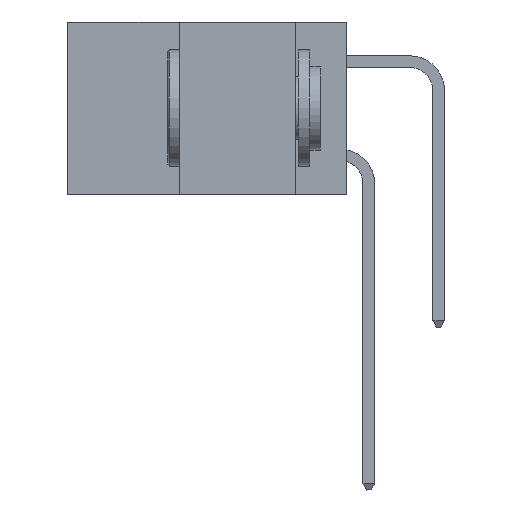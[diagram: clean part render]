
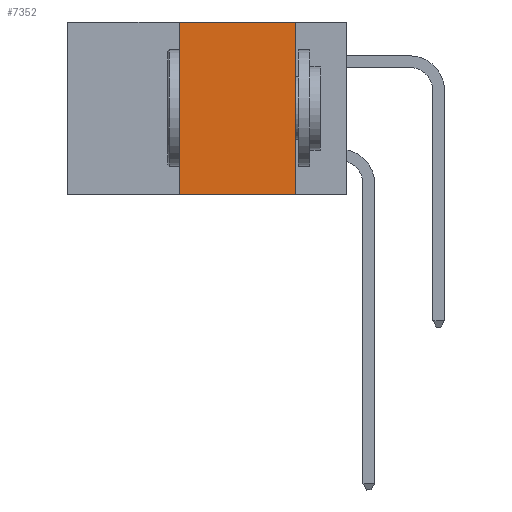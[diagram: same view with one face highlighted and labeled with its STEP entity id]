
A CAD part, left-side view. The second image highlights one B-rep face of the part: STEP entity #7352.
In plain terms, the highlighted planar face has unit normal (-1, 0, 0).
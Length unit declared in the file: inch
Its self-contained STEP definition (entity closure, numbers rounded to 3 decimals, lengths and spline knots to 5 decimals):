
#1701 = DIRECTION ( 'NONE',  ( 1., 0., 0. ) ) ;
#2170 = VERTEX_POINT ( 'NONE', #22658 ) ;
#2224 = ORIENTED_EDGE ( 'NONE', *, *, #2939, .T. ) ;
#2939 = EDGE_CURVE ( 'NONE', #2170, #36981, #4788, .T. ) ;
#4088 = CARTESIAN_POINT ( 'NONE',  ( 0., 0.6, 0. ) ) ;
#4305 = CARTESIAN_POINT ( 'NONE',  ( 0., 0.11, -0.37 ) ) ;
#4788 = LINE ( 'NONE', #7732, #15720 ) ;
#5493 = EDGE_CURVE ( 'NONE', #2170, #9404, #33022, .T. ) ;
#5904 = LINE ( 'NONE', #30891, #37155 ) ;
#6546 = EDGE_CURVE ( 'NONE', #9404, #38411, #5904, .T. ) ;
#6867 = CARTESIAN_POINT ( 'NONE',  ( 0., 0.11, 0. ) ) ;
#6978 = VECTOR ( 'NONE', #37187, 39.37008 ) ;
#7010 = DIRECTION ( 'NONE',  ( 0., -1., 0. ) ) ;
#7352 = ADVANCED_FACE ( 'NONE', ( #10082 ), #16907, .F. ) ;
#7423 = VECTOR ( 'NONE', #21959, 39.37008 ) ;
#7446 = CARTESIAN_POINT ( 'NONE',  ( 0., 0.36, 0. ) ) ;
#7732 = CARTESIAN_POINT ( 'NONE',  ( 0., 0.6, -0.37 ) ) ;
#9404 = VERTEX_POINT ( 'NONE', #7446 ) ;
#10082 = FACE_OUTER_BOUND ( 'NONE', #25897, .T. ) ;
#13397 = ORIENTED_EDGE ( 'NONE', *, *, #6546, .F. ) ;
#15720 = VECTOR ( 'NONE', #28938, 39.37008 ) ;
#16907 = PLANE ( 'NONE',  #35026 ) ;
#17008 = LINE ( 'NONE', #6867, #6978 ) ;
#17146 = CARTESIAN_POINT ( 'NONE',  ( 0., 0.11, 0. ) ) ;
#18206 = ORIENTED_EDGE ( 'NONE', *, *, #27128, .F. ) ;
#21959 = DIRECTION ( 'NONE',  ( 0., 0., 1. ) ) ;
#22658 = CARTESIAN_POINT ( 'NONE',  ( 0., 0.36, -0.37 ) ) ;
#25897 = EDGE_LOOP ( 'NONE', ( #18206, #13397, #25953, #2224 ) ) ;
#25953 = ORIENTED_EDGE ( 'NONE', *, *, #5493, .F. ) ;
#27128 = EDGE_CURVE ( 'NONE', #38411, #36981, #17008, .T. ) ;
#28938 = DIRECTION ( 'NONE',  ( 0., -1., 0. ) ) ;
#30891 = CARTESIAN_POINT ( 'NONE',  ( 0., 0.6, 0. ) ) ;
#33022 = LINE ( 'NONE', #34393, #7423 ) ;
#34393 = CARTESIAN_POINT ( 'NONE',  ( 0., 0.36, 0. ) ) ;
#35026 = AXIS2_PLACEMENT_3D ( 'NONE', #4088, #1701, #38776 ) ;
#36981 = VERTEX_POINT ( 'NONE', #4305 ) ;
#37155 = VECTOR ( 'NONE', #7010, 39.37008 ) ;
#37187 = DIRECTION ( 'NONE',  ( 0., 0., -1. ) ) ;
#38411 = VERTEX_POINT ( 'NONE', #17146 ) ;
#38776 = DIRECTION ( 'NONE',  ( 0., 0., -1. ) ) ;
